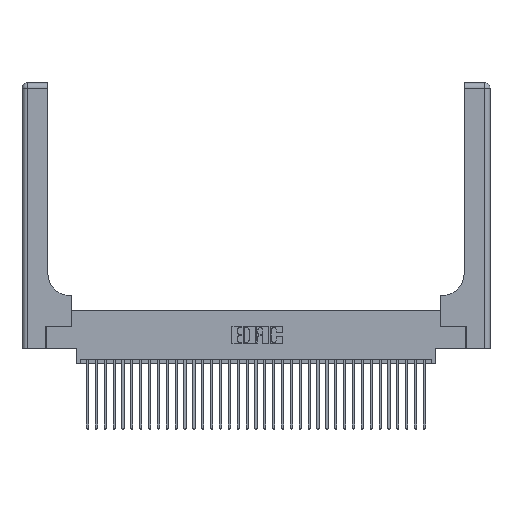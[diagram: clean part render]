
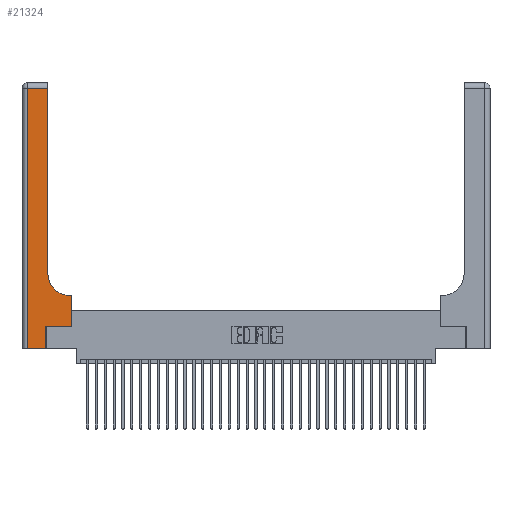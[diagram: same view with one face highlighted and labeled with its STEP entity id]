
A CAD part, top view. The second image highlights one B-rep face of the part: STEP entity #21324.
In plain terms, the highlighted planar face has unit normal (0, 0, 1).
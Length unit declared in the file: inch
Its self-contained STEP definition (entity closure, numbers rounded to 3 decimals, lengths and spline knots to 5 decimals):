
#305 = LINE ( 'NONE', #24112, #29259 ) ;
#714 = EDGE_CURVE ( 'NONE', #2131, #33159, #25288, .T. ) ;
#1189 = CARTESIAN_POINT ( 'NONE',  ( 0.2915, 0.85, 0.37 ) ) ;
#1658 = AXIS2_PLACEMENT_3D ( 'NONE', #2298, #35703, #18938 ) ;
#2131 = VERTEX_POINT ( 'NONE', #12612 ) ;
#2298 = CARTESIAN_POINT ( 'NONE',  ( 0.5415, 0.85, 0.37 ) ) ;
#2961 = ORIENTED_EDGE ( 'NONE', *, *, #29707, .T. ) ;
#3015 = CARTESIAN_POINT ( 'NONE',  ( 0.269, 0., 0.37 ) ) ;
#3313 = DIRECTION ( 'NONE',  ( -1., 0., 0. ) ) ;
#3670 = CARTESIAN_POINT ( 'NONE',  ( 0., 3., 0.37 ) ) ;
#3747 = VECTOR ( 'NONE', #20935, 39.37008 ) ;
#4200 = LINE ( 'NONE', #21137, #30552 ) ;
#6099 = VECTOR ( 'NONE', #11831, 39.37008 ) ;
#6525 = CARTESIAN_POINT ( 'NONE',  ( 0.5415, 0.6, 0.37 ) ) ;
#6906 = CARTESIAN_POINT ( 'NONE',  ( 0.5585, 0.25, 0.37 ) ) ;
#8173 = ORIENTED_EDGE ( 'NONE', *, *, #12828, .T. ) ;
#8180 = ORIENTED_EDGE ( 'NONE', *, *, #18281, .T. ) ;
#8295 = PLANE ( 'NONE',  #10750 ) ;
#8536 = VECTOR ( 'NONE', #21591, 39.37008 ) ;
#9360 = VERTEX_POINT ( 'NONE', #1189 ) ;
#9783 = CIRCLE ( 'NONE', #1658, 0.25 ) ;
#10750 = AXIS2_PLACEMENT_3D ( 'NONE', #3670, #23251, #3313 ) ;
#10874 = DIRECTION ( 'NONE',  ( 0., -1., 0. ) ) ;
#10946 = DIRECTION ( 'NONE',  ( 0., 1., 0. ) ) ;
#11038 = CARTESIAN_POINT ( 'NONE',  ( 0.06, 0., 0.37 ) ) ;
#11164 = CARTESIAN_POINT ( 'NONE',  ( 0.269, 0., 0.37 ) ) ;
#11831 = DIRECTION ( 'NONE',  ( 0., 1., 0. ) ) ;
#12154 = DIRECTION ( 'NONE',  ( -1., 0., 0. ) ) ;
#12338 = ORIENTED_EDGE ( 'NONE', *, *, #33142, .T. ) ;
#12612 = CARTESIAN_POINT ( 'NONE',  ( 0.5585, 0.6, 0.37 ) ) ;
#12828 = EDGE_CURVE ( 'NONE', #14703, #33140, #20848, .T. ) ;
#13317 = VECTOR ( 'NONE', #10946, 39.37008 ) ;
#14484 = EDGE_CURVE ( 'NONE', #33159, #9360, #9783, .T. ) ;
#14703 = VERTEX_POINT ( 'NONE', #11038 ) ;
#15262 = DIRECTION ( 'NONE',  ( 1., 0., 0. ) ) ;
#15962 = CARTESIAN_POINT ( 'NONE',  ( 0.2915, 3., 0.37 ) ) ;
#17157 = EDGE_CURVE ( 'NONE', #19867, #33362, #305, .T. ) ;
#17226 = ORIENTED_EDGE ( 'NONE', *, *, #19296, .T. ) ;
#18281 = EDGE_CURVE ( 'NONE', #31614, #14703, #4200, .T. ) ;
#18938 = DIRECTION ( 'NONE',  ( 1., 0., 0. ) ) ;
#19296 = EDGE_CURVE ( 'NONE', #9360, #28941, #26928, .T. ) ;
#19517 = CARTESIAN_POINT ( 'NONE',  ( 0.2915, 2.94, 0.37 ) ) ;
#19867 = VERTEX_POINT ( 'NONE', #21311 ) ;
#20848 = LINE ( 'NONE', #29408, #3747 ) ;
#20935 = DIRECTION ( 'NONE',  ( 1., 0., 0. ) ) ;
#21092 = EDGE_LOOP ( 'NONE', ( #17226, #12338, #8180, #8173, #2961, #22874, #32104, #34955, #32066 ) ) ;
#21137 = CARTESIAN_POINT ( 'NONE',  ( 0.06, 3., 0.37 ) ) ;
#21311 = CARTESIAN_POINT ( 'NONE',  ( 0.269, 0.25, 0.37 ) ) ;
#21324 = ADVANCED_FACE ( 'NONE', ( #30747 ), #8295, .F. ) ;
#21591 = DIRECTION ( 'NONE',  ( 0., 1., 0. ) ) ;
#22874 = ORIENTED_EDGE ( 'NONE', *, *, #17157, .T. ) ;
#23157 = LINE ( 'NONE', #31210, #6099 ) ;
#23251 = DIRECTION ( 'NONE',  ( 0., 0., -1. ) ) ;
#23293 = CARTESIAN_POINT ( 'NONE',  ( 0., 2.94, 0.37 ) ) ;
#24112 = CARTESIAN_POINT ( 'NONE',  ( 0.269, 0.25, 0.37 ) ) ;
#24853 = VECTOR ( 'NONE', #29843, 39.37008 ) ;
#25288 = LINE ( 'NONE', #31650, #24853 ) ;
#26002 = LINE ( 'NONE', #11164, #13317 ) ;
#26874 = EDGE_CURVE ( 'NONE', #33362, #2131, #23157, .T. ) ;
#26928 = LINE ( 'NONE', #15962, #8536 ) ;
#27119 = CARTESIAN_POINT ( 'NONE',  ( 0.06, 2.94, 0.37 ) ) ;
#28941 = VERTEX_POINT ( 'NONE', #19517 ) ;
#29259 = VECTOR ( 'NONE', #15262, 39.37008 ) ;
#29408 = CARTESIAN_POINT ( 'NONE',  ( 0., 0., 0.37 ) ) ;
#29707 = EDGE_CURVE ( 'NONE', #33140, #19867, #26002, .T. ) ;
#29843 = DIRECTION ( 'NONE',  ( -1., 0., 0. ) ) ;
#30552 = VECTOR ( 'NONE', #10874, 39.37008 ) ;
#30747 = FACE_OUTER_BOUND ( 'NONE', #21092, .T. ) ;
#31210 = CARTESIAN_POINT ( 'NONE',  ( 0.5585, 0.25, 0.37 ) ) ;
#31614 = VERTEX_POINT ( 'NONE', #27119 ) ;
#31650 = CARTESIAN_POINT ( 'NONE',  ( 0.2915, 0.6, 0.37 ) ) ;
#32066 = ORIENTED_EDGE ( 'NONE', *, *, #14484, .T. ) ;
#32104 = ORIENTED_EDGE ( 'NONE', *, *, #26874, .T. ) ;
#33140 = VERTEX_POINT ( 'NONE', #3015 ) ;
#33142 = EDGE_CURVE ( 'NONE', #28941, #31614, #34132, .T. ) ;
#33159 = VERTEX_POINT ( 'NONE', #6525 ) ;
#33362 = VERTEX_POINT ( 'NONE', #6906 ) ;
#34132 = LINE ( 'NONE', #23293, #35491 ) ;
#34955 = ORIENTED_EDGE ( 'NONE', *, *, #714, .T. ) ;
#35491 = VECTOR ( 'NONE', #12154, 39.37008 ) ;
#35703 = DIRECTION ( 'NONE',  ( 0., 0., -1. ) ) ;
